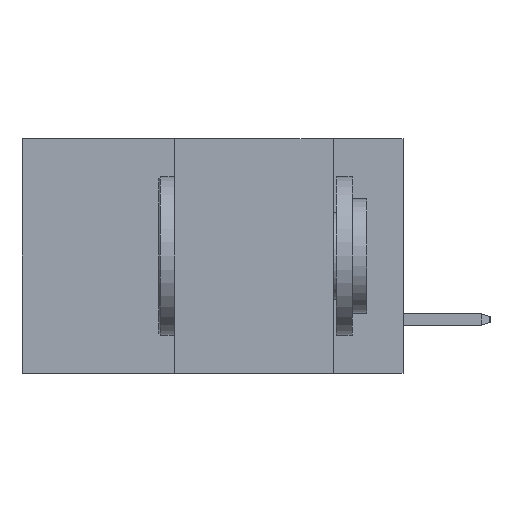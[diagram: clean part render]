
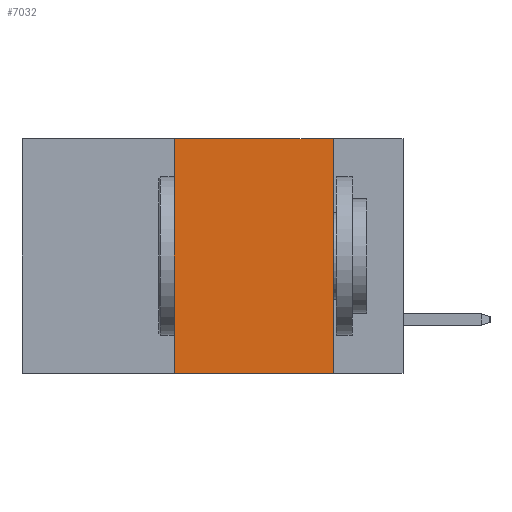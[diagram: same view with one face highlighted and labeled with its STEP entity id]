
A CAD part, left-side view. The second image highlights one B-rep face of the part: STEP entity #7032.
In plain terms, the highlighted planar face has unit normal (-1, 0, 0).
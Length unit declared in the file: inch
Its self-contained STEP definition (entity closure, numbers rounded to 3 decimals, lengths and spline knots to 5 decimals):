
#686 = EDGE_CURVE ( 'NONE', #10563, #3802, #3958, .T. ) ;
#1180 = VERTEX_POINT ( 'NONE', #10809 ) ;
#1434 = ORIENTED_EDGE ( 'NONE', *, *, #6696, .T. ) ;
#1487 = CARTESIAN_POINT ( 'NONE',  ( 0., 0.6, 0. ) ) ;
#2041 = ORIENTED_EDGE ( 'NONE', *, *, #686, .F. ) ;
#2151 = EDGE_CURVE ( 'NONE', #3802, #1180, #4299, .T. ) ;
#2445 = ORIENTED_EDGE ( 'NONE', *, *, #2151, .F. ) ;
#2945 = CARTESIAN_POINT ( 'NONE',  ( 0., 0.36, -0.37 ) ) ;
#3140 = CARTESIAN_POINT ( 'NONE',  ( 0., 0.36, 0. ) ) ;
#3802 = VERTEX_POINT ( 'NONE', #6532 ) ;
#3958 = LINE ( 'NONE', #1487, #9167 ) ;
#4057 = DIRECTION ( 'NONE',  ( 0., -1., 0. ) ) ;
#4099 = DIRECTION ( 'NONE',  ( 1., 0., 0. ) ) ;
#4299 = LINE ( 'NONE', #7653, #8165 ) ;
#4505 = VECTOR ( 'NONE', #8288, 39.37008 ) ;
#4872 = ORIENTED_EDGE ( 'NONE', *, *, #5532, .F. ) ;
#5073 = AXIS2_PLACEMENT_3D ( 'NONE', #7393, #4099, #7451 ) ;
#5532 = EDGE_CURVE ( 'NONE', #7359, #10563, #6679, .T. ) ;
#5683 = PLANE ( 'NONE',  #5073 ) ;
#5752 = LINE ( 'NONE', #9120, #4505 ) ;
#6318 = EDGE_LOOP ( 'NONE', ( #2445, #2041, #4872, #1434 ) ) ;
#6532 = CARTESIAN_POINT ( 'NONE',  ( 0., 0.11, 0. ) ) ;
#6679 = LINE ( 'NONE', #10047, #9903 ) ;
#6696 = EDGE_CURVE ( 'NONE', #7359, #1180, #5752, .T. ) ;
#7032 = ADVANCED_FACE ( 'NONE', ( #9109 ), #5683, .F. ) ;
#7359 = VERTEX_POINT ( 'NONE', #2945 ) ;
#7393 = CARTESIAN_POINT ( 'NONE',  ( 0., 0.6, 0. ) ) ;
#7427 = DIRECTION ( 'NONE',  ( 0., 0., -1. ) ) ;
#7451 = DIRECTION ( 'NONE',  ( 0., 0., -1. ) ) ;
#7653 = CARTESIAN_POINT ( 'NONE',  ( 0., 0.11, 0. ) ) ;
#8165 = VECTOR ( 'NONE', #7427, 39.37008 ) ;
#8288 = DIRECTION ( 'NONE',  ( 0., -1., 0. ) ) ;
#9109 = FACE_OUTER_BOUND ( 'NONE', #6318, .T. ) ;
#9120 = CARTESIAN_POINT ( 'NONE',  ( 0., 0.6, -0.37 ) ) ;
#9167 = VECTOR ( 'NONE', #4057, 39.37008 ) ;
#9384 = DIRECTION ( 'NONE',  ( 0., 0., 1. ) ) ;
#9903 = VECTOR ( 'NONE', #9384, 39.37008 ) ;
#10047 = CARTESIAN_POINT ( 'NONE',  ( 0., 0.36, 0. ) ) ;
#10563 = VERTEX_POINT ( 'NONE', #3140 ) ;
#10809 = CARTESIAN_POINT ( 'NONE',  ( 0., 0.11, -0.37 ) ) ;
